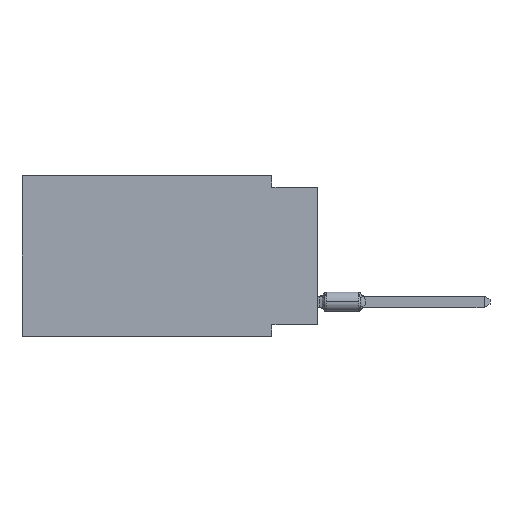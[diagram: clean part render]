
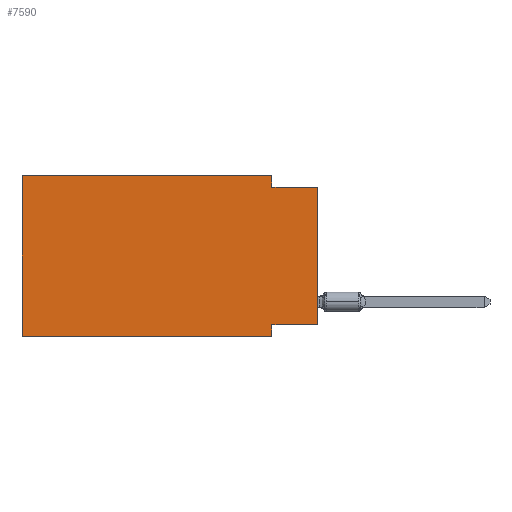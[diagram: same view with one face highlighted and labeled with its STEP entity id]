
A CAD part, left-side view. The second image highlights one B-rep face of the part: STEP entity #7590.
In plain terms, the highlighted planar face has unit normal (-1, 0, 0).
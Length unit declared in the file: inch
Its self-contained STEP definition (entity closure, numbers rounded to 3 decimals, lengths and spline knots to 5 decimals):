
#54 = EDGE_CURVE ( 'NONE', #13269, #3667, #548, .T. ) ;
#274 = CARTESIAN_POINT ( 'NONE',  ( 0., 0., 0. ) ) ;
#287 = ORIENTED_EDGE ( 'NONE', *, *, #13771, .F. ) ;
#485 = DIRECTION ( 'NONE',  ( 0., 0., -1. ) ) ;
#503 = CARTESIAN_POINT ( 'NONE',  ( 0., 0., -0.025 ) ) ;
#547 = CARTESIAN_POINT ( 'NONE',  ( 0., 0., -0.325 ) ) ;
#548 = LINE ( 'NONE', #9436, #2227 ) ;
#850 = DIRECTION ( 'NONE',  ( 0., -1., 0. ) ) ;
#1821 = ORIENTED_EDGE ( 'NONE', *, *, #7483, .F. ) ;
#2227 = VECTOR ( 'NONE', #10854, 39.37008 ) ;
#2299 = VERTEX_POINT ( 'NONE', #13513 ) ;
#2344 = DIRECTION ( 'NONE',  ( 0., 0., -1. ) ) ;
#3021 = LINE ( 'NONE', #274, #13043 ) ;
#3246 = CARTESIAN_POINT ( 'NONE',  ( 0., 0.1, -0.35 ) ) ;
#3344 = CARTESIAN_POINT ( 'NONE',  ( 0., 0.1, -0.325 ) ) ;
#3582 = CARTESIAN_POINT ( 'NONE',  ( 0., 0.1, -0.025 ) ) ;
#3667 = VERTEX_POINT ( 'NONE', #14182 ) ;
#3937 = LINE ( 'NONE', #6182, #9807 ) ;
#3941 = DIRECTION ( 'NONE',  ( 0., 0., -1. ) ) ;
#4007 = ORIENTED_EDGE ( 'NONE', *, *, #14505, .F. ) ;
#4278 = VERTEX_POINT ( 'NONE', #503 ) ;
#4533 = VECTOR ( 'NONE', #12441, 39.37008 ) ;
#4611 = VERTEX_POINT ( 'NONE', #3582 ) ;
#4793 = LINE ( 'NONE', #7063, #13341 ) ;
#4815 = CARTESIAN_POINT ( 'NONE',  ( 0., 0.645, 0. ) ) ;
#5727 = AXIS2_PLACEMENT_3D ( 'NONE', #15075, #8725, #2344 ) ;
#6182 = CARTESIAN_POINT ( 'NONE',  ( 0., 0.645, 0. ) ) ;
#6193 = PLANE ( 'NONE',  #5727 ) ;
#6488 = ORIENTED_EDGE ( 'NONE', *, *, #12015, .F. ) ;
#6943 = VERTEX_POINT ( 'NONE', #547 ) ;
#7063 = CARTESIAN_POINT ( 'NONE',  ( 0., 0., -0.025 ) ) ;
#7219 = LINE ( 'NONE', #9660, #12942 ) ;
#7483 = EDGE_CURVE ( 'NONE', #6943, #9110, #7219, .T. ) ;
#7502 = LINE ( 'NONE', #9930, #4533 ) ;
#7590 = ADVANCED_FACE ( 'NONE', ( #8631 ), #6193, .F. ) ;
#8134 = DIRECTION ( 'NONE',  ( 0., 0., 1. ) ) ;
#8271 = VECTOR ( 'NONE', #3941, 39.37008 ) ;
#8631 = FACE_OUTER_BOUND ( 'NONE', #12949, .T. ) ;
#8725 = DIRECTION ( 'NONE',  ( 1., 0., 0. ) ) ;
#8975 = DIRECTION ( 'NONE',  ( 0., 1., 0. ) ) ;
#9110 = VERTEX_POINT ( 'NONE', #3344 ) ;
#9429 = ORIENTED_EDGE ( 'NONE', *, *, #16392, .F. ) ;
#9436 = CARTESIAN_POINT ( 'NONE',  ( 0., 0.645, -0.35 ) ) ;
#9660 = CARTESIAN_POINT ( 'NONE',  ( 0., 0., -0.325 ) ) ;
#9807 = VECTOR ( 'NONE', #12881, 39.37008 ) ;
#9930 = CARTESIAN_POINT ( 'NONE',  ( 0., 0.645, 0. ) ) ;
#10056 = ORIENTED_EDGE ( 'NONE', *, *, #54, .T. ) ;
#10642 = CARTESIAN_POINT ( 'NONE',  ( 0., 0.1, 0. ) ) ;
#10854 = DIRECTION ( 'NONE',  ( 0., -1., 0. ) ) ;
#11197 = VECTOR ( 'NONE', #485, 39.37008 ) ;
#11719 = ORIENTED_EDGE ( 'NONE', *, *, #16195, .F. ) ;
#11803 = CARTESIAN_POINT ( 'NONE',  ( 0., 0.645, -0.35 ) ) ;
#12015 = EDGE_CURVE ( 'NONE', #13269, #14621, #3937, .T. ) ;
#12441 = DIRECTION ( 'NONE',  ( 0., -1., 0. ) ) ;
#12881 = DIRECTION ( 'NONE',  ( 0., 0., 1. ) ) ;
#12942 = VECTOR ( 'NONE', #8975, 39.37008 ) ;
#12949 = EDGE_LOOP ( 'NONE', ( #15242, #287, #4007, #9429, #6488, #10056, #11719, #1821 ) ) ;
#13043 = VECTOR ( 'NONE', #8134, 39.37008 ) ;
#13144 = LINE ( 'NONE', #10642, #8271 ) ;
#13269 = VERTEX_POINT ( 'NONE', #11803 ) ;
#13341 = VECTOR ( 'NONE', #850, 39.37008 ) ;
#13513 = CARTESIAN_POINT ( 'NONE',  ( 0., 0.1, 0. ) ) ;
#13624 = LINE ( 'NONE', #3246, #11197 ) ;
#13771 = EDGE_CURVE ( 'NONE', #4611, #4278, #4793, .T. ) ;
#14182 = CARTESIAN_POINT ( 'NONE',  ( 0., 0.1, -0.35 ) ) ;
#14505 = EDGE_CURVE ( 'NONE', #2299, #4611, #13144, .T. ) ;
#14621 = VERTEX_POINT ( 'NONE', #4815 ) ;
#15075 = CARTESIAN_POINT ( 'NONE',  ( 0., 0.645, 0. ) ) ;
#15224 = EDGE_CURVE ( 'NONE', #6943, #4278, #3021, .T. ) ;
#15242 = ORIENTED_EDGE ( 'NONE', *, *, #15224, .T. ) ;
#16195 = EDGE_CURVE ( 'NONE', #9110, #3667, #13624, .T. ) ;
#16392 = EDGE_CURVE ( 'NONE', #14621, #2299, #7502, .T. ) ;
